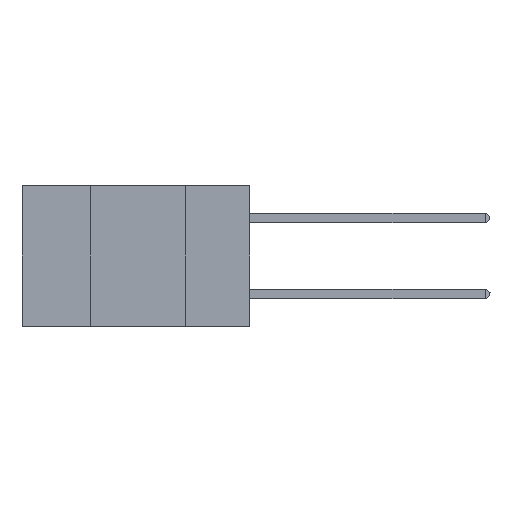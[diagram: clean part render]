
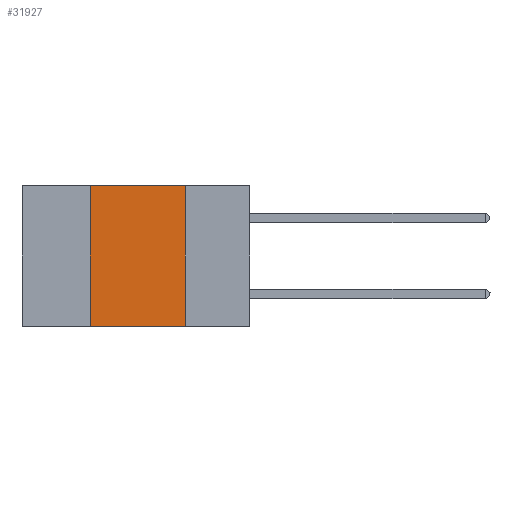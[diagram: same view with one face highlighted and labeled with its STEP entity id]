
A CAD part, left-side view. The second image highlights one B-rep face of the part: STEP entity #31927.
In plain terms, the highlighted planar face has unit normal (-1, 0, 0).
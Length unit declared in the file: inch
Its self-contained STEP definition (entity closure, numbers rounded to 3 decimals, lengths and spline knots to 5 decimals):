
#178 = PLANE ( 'NONE',  #25428 ) ;
#534 = LINE ( 'NONE', #10684, #16833 ) ;
#1607 = EDGE_CURVE ( 'NONE', #8943, #24069, #18145, .T. ) ;
#2347 = FACE_OUTER_BOUND ( 'NONE', #7803, .T. ) ;
#4016 = DIRECTION ( 'NONE',  ( 0., 0., 1. ) ) ;
#4598 = ORIENTED_EDGE ( 'NONE', *, *, #19172, .F. ) ;
#4677 = LINE ( 'NONE', #24350, #5723 ) ;
#4679 = DIRECTION ( 'NONE',  ( 0., 0., -1. ) ) ;
#5723 = VECTOR ( 'NONE', #4016, 39.37008 ) ;
#5806 = VERTEX_POINT ( 'NONE', #8255 ) ;
#6401 = CARTESIAN_POINT ( 'NONE',  ( 0., 0.42, 0. ) ) ;
#6605 = LINE ( 'NONE', #27413, #30419 ) ;
#6708 = ORIENTED_EDGE ( 'NONE', *, *, #1607, .T. ) ;
#7803 = EDGE_LOOP ( 'NONE', ( #4598, #17349, #19818, #6708 ) ) ;
#8255 = CARTESIAN_POINT ( 'NONE',  ( 0., 0.17, 0. ) ) ;
#8943 = VERTEX_POINT ( 'NONE', #30938 ) ;
#10332 = CARTESIAN_POINT ( 'NONE',  ( 0., 0.6, 0. ) ) ;
#10684 = CARTESIAN_POINT ( 'NONE',  ( 0., 0.17, 0. ) ) ;
#12599 = VECTOR ( 'NONE', #20175, 39.37008 ) ;
#16833 = VECTOR ( 'NONE', #20854, 39.37008 ) ;
#17349 = ORIENTED_EDGE ( 'NONE', *, *, #21714, .F. ) ;
#18145 = LINE ( 'NONE', #22675, #12599 ) ;
#19172 = EDGE_CURVE ( 'NONE', #5806, #24069, #534, .T. ) ;
#19818 = ORIENTED_EDGE ( 'NONE', *, *, #31317, .F. ) ;
#20175 = DIRECTION ( 'NONE',  ( 0., -1., 0. ) ) ;
#20854 = DIRECTION ( 'NONE',  ( 0., 0., -1. ) ) ;
#21714 = EDGE_CURVE ( 'NONE', #22106, #5806, #6605, .T. ) ;
#22106 = VERTEX_POINT ( 'NONE', #6401 ) ;
#22675 = CARTESIAN_POINT ( 'NONE',  ( 0., 0.6, -0.37 ) ) ;
#24069 = VERTEX_POINT ( 'NONE', #29737 ) ;
#24350 = CARTESIAN_POINT ( 'NONE',  ( 0., 0.42, 0. ) ) ;
#25169 = DIRECTION ( 'NONE',  ( 1., 0., 0. ) ) ;
#25428 = AXIS2_PLACEMENT_3D ( 'NONE', #10332, #25169, #4679 ) ;
#27413 = CARTESIAN_POINT ( 'NONE',  ( 0., 0.6, 0. ) ) ;
#29737 = CARTESIAN_POINT ( 'NONE',  ( 0., 0.17, -0.37 ) ) ;
#29898 = DIRECTION ( 'NONE',  ( 0., -1., 0. ) ) ;
#30419 = VECTOR ( 'NONE', #29898, 39.37008 ) ;
#30938 = CARTESIAN_POINT ( 'NONE',  ( 0., 0.42, -0.37 ) ) ;
#31317 = EDGE_CURVE ( 'NONE', #8943, #22106, #4677, .T. ) ;
#31927 = ADVANCED_FACE ( 'NONE', ( #2347 ), #178, .F. ) ;
